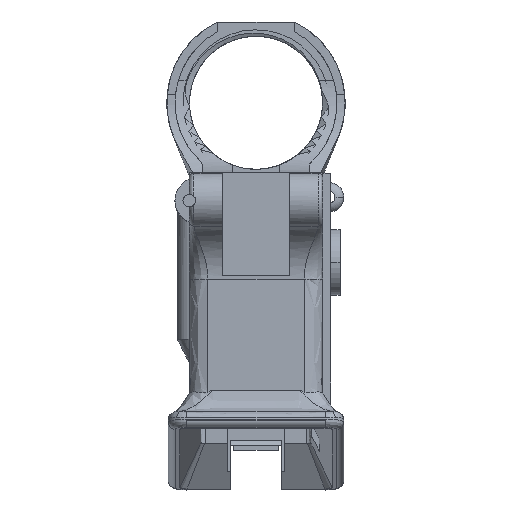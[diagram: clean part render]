
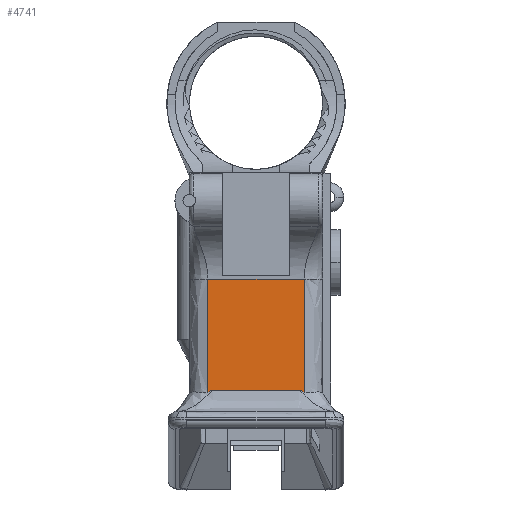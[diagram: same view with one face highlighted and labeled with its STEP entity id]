
A CAD part, top view. The second image highlights one B-rep face of the part: STEP entity #4741.
In plain terms, the highlighted planar face has unit normal (0, 0, 1).
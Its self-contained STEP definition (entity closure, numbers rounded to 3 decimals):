
#1490 = CARTESIAN_POINT ( 'NONE',  ( 10.25, -22.658, 67. ) ) ;
#1925 = CARTESIAN_POINT ( 'NONE',  ( 9.293, -46.365, 67. ) ) ;
#2080 = CARTESIAN_POINT ( 'NONE',  ( -9.578, -46.439, 67. ) ) ;
#2319 = CARTESIAN_POINT ( 'NONE',  ( -9.671, -46.474, 67. ) ) ;
#2440 = CARTESIAN_POINT ( 'NONE',  ( -9.734, -46.499, 67. ) ) ;
#2521 = CARTESIAN_POINT ( 'NONE',  ( 9.577, -46.438, 67. ) ) ;
#3390 = DIRECTION ( 'NONE',  ( 1., 0., 0. ) ) ;
#3607 = CARTESIAN_POINT ( 'NONE',  ( -10.25, -22.658, 67. ) ) ;
#3650 = CARTESIAN_POINT ( 'NONE',  ( 10.25, -46.601, 67. ) ) ;
#4717 = CARTESIAN_POINT ( 'NONE',  ( 9.342, -46.365, 67. ) ) ;
#4741 = ADVANCED_FACE ( 'NONE', ( #17463 ), #26723, .T. ) ;
#5086 = VERTEX_POINT ( 'NONE', #14242 ) ;
#5103 = CARTESIAN_POINT ( 'NONE',  ( -9.785, -46.52, 67. ) ) ;
#5226 = CARTESIAN_POINT ( 'NONE',  ( -9.341, -46.365, 67. ) ) ;
#5304 = CARTESIAN_POINT ( 'NONE',  ( 9.768, -46.513, 67. ) ) ;
#5539 = CARTESIAN_POINT ( 'NONE',  ( 9.555, -46.43, 67. ) ) ;
#7928 = CARTESIAN_POINT ( 'NONE',  ( 9.651, -46.466, 67. ) ) ;
#8153 = CARTESIAN_POINT ( 'NONE',  ( -11.35, -22.658, 67. ) ) ;
#8164 = CARTESIAN_POINT ( 'NONE',  ( 9.776, -46.516, 67. ) ) ;
#8954 = CARTESIAN_POINT ( 'NONE',  ( 10.25, -46.483, 67. ) ) ;
#8959 = ORIENTED_EDGE ( 'NONE', *, *, #16738, .F. ) ;
#9158 = CARTESIAN_POINT ( 'NONE',  ( -10.25, -38.463, 67. ) ) ;
#9266 = CARTESIAN_POINT ( 'NONE',  ( -10.25, -22.658, 67. ) ) ;
#9606 = ORIENTED_EDGE ( 'NONE', *, *, #30104, .T. ) ;
#10397 = CARTESIAN_POINT ( 'NONE',  ( -10.026, -46.622, 67. ) ) ;
#11377 = B_SPLINE_CURVE_WITH_KNOTS ( 'NONE', 3,
 ( #24202, #35644, #10397, #15945, #18713, #27235, #18826, #13161, #5103, #2440, #2319, #18594, #18952, #21738, #2080, #30172, #21623, #5226, #13517 ),
 .UNSPECIFIED., .F., .F.,
 ( 4, 1, 1, 1, 1, 2, 2, 1, 2, 2, 1, 1, 4 ),
 ( 0., 0.25, 0.375, 0.437, 0.469, 0.484, 0.5, 0.625, 0.687, 0.703, 0.719, 0.75, 1. ),
 .UNSPECIFIED. ) ;
#13161 = CARTESIAN_POINT ( 'NONE',  ( -9.787, -46.521, 67. ) ) ;
#13174 = CARTESIAN_POINT ( 'NONE',  ( 14.25, -46.365, 67. ) ) ;
#13203 = B_SPLINE_CURVE_WITH_KNOTS ( 'NONE', 3,
 ( #25911, #3650, #8954, #25554, #34321, #33962, #23109 ),
 .UNSPECIFIED., .F., .F.,
 ( 4, 3, 4 ),
 ( 0.049, 0.05, 0.073 ),
 .UNSPECIFIED. ) ;
#13517 = CARTESIAN_POINT ( 'NONE',  ( -9.293, -46.365, 67. ) ) ;
#13590 = DIRECTION ( 'NONE',  ( 0., 0., 1. ) ) ;
#13711 = DIRECTION ( 'NONE',  ( 0., -1., 0. ) ) ;
#13721 = CARTESIAN_POINT ( 'NONE',  ( 9.43, -46.386, 67. ) ) ;
#14242 = CARTESIAN_POINT ( 'NONE',  ( -10.25, -46.719, 67. ) ) ;
#14773 = CARTESIAN_POINT ( 'NONE',  ( 9.293, -46.365, 67. ) ) ;
#15945 = CARTESIAN_POINT ( 'NONE',  ( -9.896, -46.566, 67. ) ) ;
#16251 = CARTESIAN_POINT ( 'NONE',  ( 9.74, -46.502, 67. ) ) ;
#16369 = CARTESIAN_POINT ( 'NONE',  ( 10.061, -46.636, 67. ) ) ;
#16738 = EDGE_CURVE ( 'NONE', #30032, #18374, #20121, .T. ) ;
#17347 = CARTESIAN_POINT ( 'NONE',  ( -10.25, -30.56, 67. ) ) ;
#17463 = FACE_OUTER_BOUND ( 'NONE', #32506, .T. ) ;
#17489 = CARTESIAN_POINT ( 'NONE',  ( -11.35, -22.658, 67. ) ) ;
#18374 = VERTEX_POINT ( 'NONE', #20668 ) ;
#18594 = CARTESIAN_POINT ( 'NONE',  ( -9.616, -46.453, 67. ) ) ;
#18713 = CARTESIAN_POINT ( 'NONE',  ( -9.836, -46.541, 67. ) ) ;
#18774 = AXIS2_PLACEMENT_3D ( 'NONE', #8153, #13590, #13711 ) ;
#18826 = CARTESIAN_POINT ( 'NONE',  ( -9.795, -46.524, 67. ) ) ;
#18865 = ORIENTED_EDGE ( 'NONE', *, *, #24659, .T. ) ;
#18952 = CARTESIAN_POINT ( 'NONE',  ( -9.595, -46.445, 67. ) ) ;
#19097 = LINE ( 'NONE', #17489, #31359 ) ;
#20087 = EDGE_CURVE ( 'NONE', #20616, #23737, #19097, .T. ) ;
#20121 = LINE ( 'NONE', #13174, #21394 ) ;
#20616 = VERTEX_POINT ( 'NONE', #3607 ) ;
#20668 = CARTESIAN_POINT ( 'NONE',  ( -9.293, -46.365, 67. ) ) ;
#21394 = VECTOR ( 'NONE', #24339, 1000. ) ;
#21463 = EDGE_CURVE ( 'NONE', #20616, #5086, #34992, .T. ) ;
#21476 = VERTEX_POINT ( 'NONE', #25746 ) ;
#21623 = CARTESIAN_POINT ( 'NONE',  ( -9.427, -46.385, 67. ) ) ;
#21705 = CARTESIAN_POINT ( 'NONE',  ( 9.61, -46.451, 67. ) ) ;
#21738 = CARTESIAN_POINT ( 'NONE',  ( -9.592, -46.444, 67. ) ) ;
#22937 = CARTESIAN_POINT ( 'NONE',  ( -10.25, -46.483, 67. ) ) ;
#23109 = CARTESIAN_POINT ( 'NONE',  ( 10.25, -22.658, 67. ) ) ;
#23737 = VERTEX_POINT ( 'NONE', #1490 ) ;
#24202 = CARTESIAN_POINT ( 'NONE',  ( -10.25, -46.719, 67. ) ) ;
#24339 = DIRECTION ( 'NONE',  ( -1., 0., 0. ) ) ;
#24510 = CARTESIAN_POINT ( 'NONE',  ( 9.757, -46.509, 67. ) ) ;
#24659 = EDGE_CURVE ( 'NONE', #5086, #18374, #11377, .T. ) ;
#24755 = CARTESIAN_POINT ( 'NONE',  ( 9.581, -46.44, 67. ) ) ;
#25006 = CARTESIAN_POINT ( 'NONE',  ( 9.702, -46.487, 67. ) ) ;
#25554 = CARTESIAN_POINT ( 'NONE',  ( 10.25, -46.365, 67. ) ) ;
#25746 = CARTESIAN_POINT ( 'NONE',  ( 10.25, -46.719, 67. ) ) ;
#25911 = CARTESIAN_POINT ( 'NONE',  ( 10.25, -46.719, 67. ) ) ;
#26481 = ORIENTED_EDGE ( 'NONE', *, *, #26763, .T. ) ;
#26723 = PLANE ( 'NONE',  #18774 ) ;
#26763 = EDGE_CURVE ( 'NONE', #30032, #21476, #34532, .T. ) ;
#26850 = ORIENTED_EDGE ( 'NONE', *, *, #21463, .T. ) ;
#27235 = CARTESIAN_POINT ( 'NONE',  ( -9.807, -46.529, 67. ) ) ;
#27682 = CARTESIAN_POINT ( 'NONE',  ( 9.589, -46.443, 67. ) ) ;
#28439 = ORIENTED_EDGE ( 'NONE', *, *, #20087, .F. ) ;
#28561 = CARTESIAN_POINT ( 'NONE',  ( -10.25, -46.719, 67. ) ) ;
#28688 = CARTESIAN_POINT ( 'NONE',  ( -10.25, -46.601, 67. ) ) ;
#30032 = VERTEX_POINT ( 'NONE', #14773 ) ;
#30104 = EDGE_CURVE ( 'NONE', #21476, #23737, #13203, .T. ) ;
#30133 = CARTESIAN_POINT ( 'NONE',  ( 10.25, -46.719, 67. ) ) ;
#30172 = CARTESIAN_POINT ( 'NONE',  ( -9.556, -46.431, 67. ) ) ;
#31359 = VECTOR ( 'NONE', #3390, 1000. ) ;
#32506 = EDGE_LOOP ( 'NONE', ( #28439, #26850, #18865, #8959, #26481, #9606 ) ) ;
#33914 = CARTESIAN_POINT ( 'NONE',  ( -10.25, -46.365, 67. ) ) ;
#33962 = CARTESIAN_POINT ( 'NONE',  ( 10.25, -30.56, 67. ) ) ;
#34321 = CARTESIAN_POINT ( 'NONE',  ( 10.25, -38.463, 67. ) ) ;
#34532 = B_SPLINE_CURVE_WITH_KNOTS ( 'NONE', 3,
 ( #1925, #4717, #13721, #5539, #2521, #24755, #27682, #21705, #7928, #25006, #16251, #24510, #5304, #8164, #35959, #16369, #30133 ),
 .UNSPECIFIED., .F., .F.,
 ( 4, 1, 2, 2, 1, 1, 1, 1, 2, 2, 4 ),
 ( 0., 0.25, 0.281, 0.297, 0.313, 0.375, 0.438, 0.469, 0.484, 0.5, 1. ),
 .UNSPECIFIED. ) ;
#34992 = B_SPLINE_CURVE_WITH_KNOTS ( 'NONE', 3,
 ( #9266, #17347, #9158, #33914, #22937, #28688, #28561 ),
 .UNSPECIFIED., .F., .F.,
 ( 4, 3, 4 ),
 ( 0., 0.024, 0.024 ),
 .UNSPECIFIED. ) ;
#35644 = CARTESIAN_POINT ( 'NONE',  ( -10.156, -46.678, 67. ) ) ;
#35959 = CARTESIAN_POINT ( 'NONE',  ( 9.905, -46.569, 67. ) ) ;
